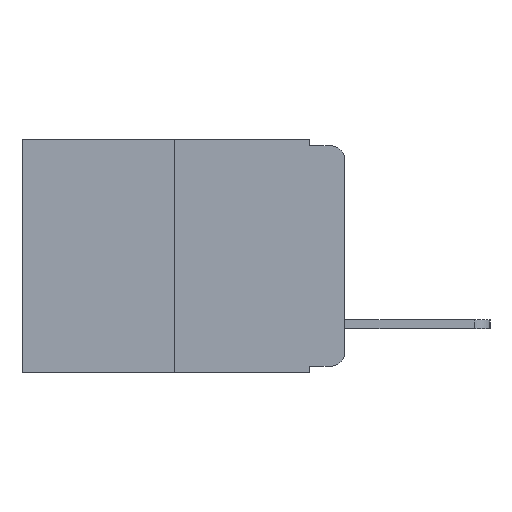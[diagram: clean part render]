
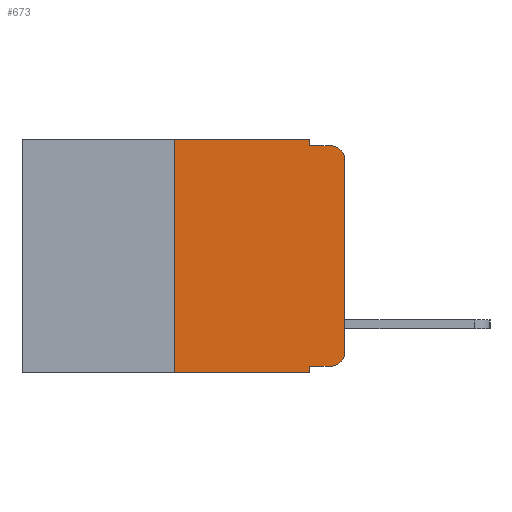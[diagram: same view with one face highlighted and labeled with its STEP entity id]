
A CAD part, left-side view. The second image highlights one B-rep face of the part: STEP entity #673.
In plain terms, the highlighted planar face has unit normal (-1, 0, 0).
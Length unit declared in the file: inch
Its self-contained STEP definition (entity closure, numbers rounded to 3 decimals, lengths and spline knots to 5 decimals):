
#223 = ORIENTED_EDGE ( 'NONE', *, *, #3206, .T. ) ;
#461 = CIRCLE ( 'NONE', #17221, 0.02 ) ;
#552 = LINE ( 'NONE', #19091, #8470 ) ;
#673 = ADVANCED_FACE ( 'NONE', ( #7310 ), #8897, .F. ) ;
#866 = EDGE_CURVE ( 'NONE', #9976, #6227, #15707, .T. ) ;
#901 = DIRECTION ( 'NONE',  ( 0., 0., 1. ) ) ;
#1222 = LINE ( 'NONE', #19466, #13711 ) ;
#1312 = LINE ( 'NONE', #10391, #16436 ) ;
#1844 = DIRECTION ( 'NONE',  ( 0., -1., 0. ) ) ;
#2712 = LINE ( 'NONE', #19721, #14669 ) ;
#2813 = VECTOR ( 'NONE', #1844, 39.37008 ) ;
#2824 = VERTEX_POINT ( 'NONE', #17239 ) ;
#2929 = EDGE_CURVE ( 'NONE', #10832, #6227, #3457, .T. ) ;
#2970 = VECTOR ( 'NONE', #6764, 39.37008 ) ;
#3027 = CIRCLE ( 'NONE', #10410, 0.02 ) ;
#3206 = EDGE_CURVE ( 'NONE', #10832, #5344, #2712, .T. ) ;
#3365 = LINE ( 'NONE', #9838, #14353 ) ;
#3457 = LINE ( 'NONE', #17507, #2970 ) ;
#3610 = CARTESIAN_POINT ( 'NONE',  ( 0., 0.02, -0.313 ) ) ;
#3611 = CARTESIAN_POINT ( 'NONE',  ( 0., 0.051, -0.333 ) ) ;
#3754 = DIRECTION ( 'NONE',  ( -1., 0., 0. ) ) ;
#4428 = ORIENTED_EDGE ( 'NONE', *, *, #14815, .T. ) ;
#4710 = EDGE_CURVE ( 'NONE', #5344, #9753, #461, .T. ) ;
#5202 = ORIENTED_EDGE ( 'NONE', *, *, #17130, .F. ) ;
#5246 = DIRECTION ( 'NONE',  ( 0., 0., -1. ) ) ;
#5307 = VERTEX_POINT ( 'NONE', #18998 ) ;
#5344 = VERTEX_POINT ( 'NONE', #17484 ) ;
#5794 = VERTEX_POINT ( 'NONE', #11329 ) ;
#6157 = CARTESIAN_POINT ( 'NONE',  ( 0., 0.25, 0. ) ) ;
#6227 = VERTEX_POINT ( 'NONE', #9264 ) ;
#6342 = CARTESIAN_POINT ( 'NONE',  ( 0., 0., -0.313 ) ) ;
#6693 = ORIENTED_EDGE ( 'NONE', *, *, #866, .T. ) ;
#6764 = DIRECTION ( 'NONE',  ( 0., 0., -1. ) ) ;
#6862 = CARTESIAN_POINT ( 'NONE',  ( 0., 0.25, -0.343 ) ) ;
#6976 = CARTESIAN_POINT ( 'NONE',  ( 0., 0.051, -0.01 ) ) ;
#6984 = EDGE_LOOP ( 'NONE', ( #4428, #19142, #7413, #5202, #13938, #17979, #6693, #16327, #223, #16813 ) ) ;
#7310 = FACE_OUTER_BOUND ( 'NONE', #6984, .T. ) ;
#7413 = ORIENTED_EDGE ( 'NONE', *, *, #11765, .F. ) ;
#7511 = DIRECTION ( 'NONE',  ( 0., -1., 0. ) ) ;
#8470 = VECTOR ( 'NONE', #8481, 39.37008 ) ;
#8481 = DIRECTION ( 'NONE',  ( 0., -1., 0. ) ) ;
#8722 = EDGE_CURVE ( 'NONE', #13610, #5307, #552, .T. ) ;
#8897 = PLANE ( 'NONE',  #13872 ) ;
#8942 = DIRECTION ( 'NONE',  ( 0., 0., -1. ) ) ;
#9264 = CARTESIAN_POINT ( 'NONE',  ( 0., 0.051, -0.343 ) ) ;
#9753 = VERTEX_POINT ( 'NONE', #6342 ) ;
#9838 = CARTESIAN_POINT ( 'NONE',  ( 0., 0.051, 0. ) ) ;
#9976 = VERTEX_POINT ( 'NONE', #6862 ) ;
#10391 = CARTESIAN_POINT ( 'NONE',  ( 0., 0.25, 0. ) ) ;
#10410 = AXIS2_PLACEMENT_3D ( 'NONE', #13115, #3754, #14645 ) ;
#10832 = VERTEX_POINT ( 'NONE', #3611 ) ;
#10896 = LINE ( 'NONE', #6976, #18523 ) ;
#11329 = CARTESIAN_POINT ( 'NONE',  ( 0., 0.051, -0.01 ) ) ;
#11740 = EDGE_CURVE ( 'NONE', #17218, #2824, #3027, .T. ) ;
#11765 = EDGE_CURVE ( 'NONE', #5794, #2824, #10896, .T. ) ;
#11944 = DIRECTION ( 'NONE',  ( 0., 0., 1. ) ) ;
#13115 = CARTESIAN_POINT ( 'NONE',  ( 0., 0.02, -0.03 ) ) ;
#13610 = VERTEX_POINT ( 'NONE', #6157 ) ;
#13711 = VECTOR ( 'NONE', #901, 39.37008 ) ;
#13872 = AXIS2_PLACEMENT_3D ( 'NONE', #19226, #19664, #8942 ) ;
#13938 = ORIENTED_EDGE ( 'NONE', *, *, #8722, .F. ) ;
#14353 = VECTOR ( 'NONE', #18983, 39.37008 ) ;
#14520 = DIRECTION ( 'NONE',  ( -1., 0., 0. ) ) ;
#14645 = DIRECTION ( 'NONE',  ( 0., 0., -1. ) ) ;
#14669 = VECTOR ( 'NONE', #7511, 39.37008 ) ;
#14815 = EDGE_CURVE ( 'NONE', #9753, #17218, #1222, .T. ) ;
#15707 = LINE ( 'NONE', #17923, #2813 ) ;
#16215 = CARTESIAN_POINT ( 'NONE',  ( 0., 0., -0.03 ) ) ;
#16327 = ORIENTED_EDGE ( 'NONE', *, *, #2929, .F. ) ;
#16436 = VECTOR ( 'NONE', #11944, 39.37008 ) ;
#16813 = ORIENTED_EDGE ( 'NONE', *, *, #4710, .T. ) ;
#17130 = EDGE_CURVE ( 'NONE', #5307, #5794, #3365, .T. ) ;
#17218 = VERTEX_POINT ( 'NONE', #16215 ) ;
#17221 = AXIS2_PLACEMENT_3D ( 'NONE', #3610, #14520, #5246 ) ;
#17239 = CARTESIAN_POINT ( 'NONE',  ( 0., 0.02, -0.01 ) ) ;
#17484 = CARTESIAN_POINT ( 'NONE',  ( 0., 0.02, -0.333 ) ) ;
#17507 = CARTESIAN_POINT ( 'NONE',  ( 0., 0.051, 0. ) ) ;
#17711 = DIRECTION ( 'NONE',  ( 0., -1., 0. ) ) ;
#17923 = CARTESIAN_POINT ( 'NONE',  ( 0., 0.473, -0.343 ) ) ;
#17979 = ORIENTED_EDGE ( 'NONE', *, *, #18876, .F. ) ;
#18523 = VECTOR ( 'NONE', #17711, 39.37008 ) ;
#18876 = EDGE_CURVE ( 'NONE', #9976, #13610, #1312, .T. ) ;
#18983 = DIRECTION ( 'NONE',  ( 0., 0., -1. ) ) ;
#18998 = CARTESIAN_POINT ( 'NONE',  ( 0., 0.051, 0. ) ) ;
#19091 = CARTESIAN_POINT ( 'NONE',  ( 0., 0.473, 0. ) ) ;
#19142 = ORIENTED_EDGE ( 'NONE', *, *, #11740, .T. ) ;
#19226 = CARTESIAN_POINT ( 'NONE',  ( 0., 0.473, 0. ) ) ;
#19466 = CARTESIAN_POINT ( 'NONE',  ( 0., 0., 0. ) ) ;
#19664 = DIRECTION ( 'NONE',  ( 1., 0., 0. ) ) ;
#19721 = CARTESIAN_POINT ( 'NONE',  ( 0., 0.051, -0.333 ) ) ;
